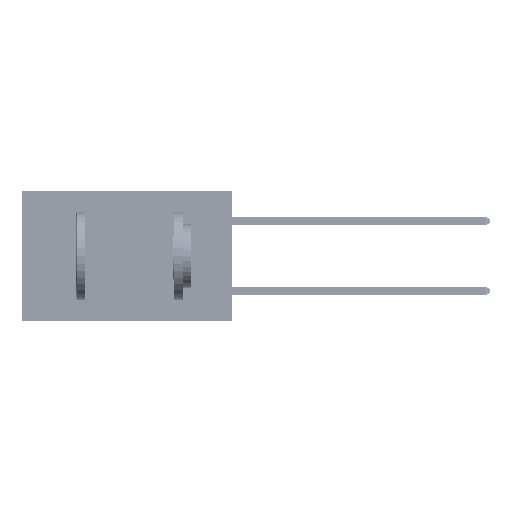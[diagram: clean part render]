
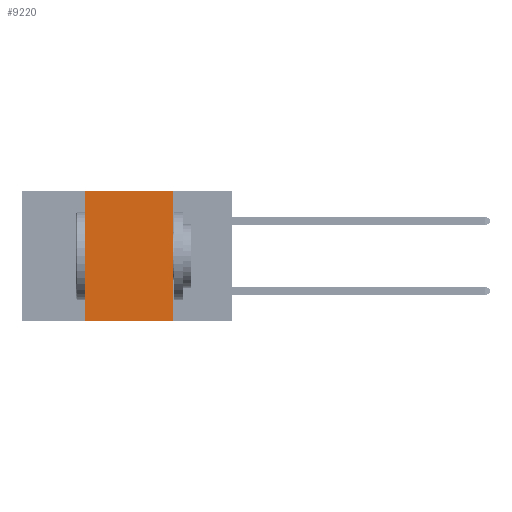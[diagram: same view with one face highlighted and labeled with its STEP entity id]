
A CAD part, left-side view. The second image highlights one B-rep face of the part: STEP entity #9220.
In plain terms, the highlighted planar face has unit normal (-1, 0, 0).
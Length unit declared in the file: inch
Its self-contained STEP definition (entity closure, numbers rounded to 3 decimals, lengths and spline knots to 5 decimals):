
#610 = DIRECTION ( 'NONE',  ( 0., 0., -1. ) ) ;
#2530 = EDGE_CURVE ( 'NONE', #25700, #29957, #48167, .T. ) ;
#3444 = ORIENTED_EDGE ( 'NONE', *, *, #2530, .F. ) ;
#4297 = CARTESIAN_POINT ( 'NONE',  ( 0., 0.17, 0. ) ) ;
#7742 = DIRECTION ( 'NONE',  ( 0., -1., 0. ) ) ;
#7837 = EDGE_CURVE ( 'NONE', #26606, #25754, #17936, .T. ) ;
#9220 = ADVANCED_FACE ( 'NONE', ( #38827 ), #36111, .F. ) ;
#11844 = CARTESIAN_POINT ( 'NONE',  ( 0., 0.6, 0. ) ) ;
#13499 = LINE ( 'NONE', #45412, #21507 ) ;
#13538 = LINE ( 'NONE', #27073, #37643 ) ;
#14273 = CARTESIAN_POINT ( 'NONE',  ( 0., 0.42, 0. ) ) ;
#16411 = CARTESIAN_POINT ( 'NONE',  ( 0., 0.6, 0. ) ) ;
#17936 = LINE ( 'NONE', #32562, #32739 ) ;
#21033 = DIRECTION ( 'NONE',  ( 0., -1., 0. ) ) ;
#21507 = VECTOR ( 'NONE', #33598, 39.37008 ) ;
#25700 = VERTEX_POINT ( 'NONE', #14273 ) ;
#25754 = VERTEX_POINT ( 'NONE', #38962 ) ;
#26606 = VERTEX_POINT ( 'NONE', #27355 ) ;
#27073 = CARTESIAN_POINT ( 'NONE',  ( 0., 0.42, 0. ) ) ;
#27355 = CARTESIAN_POINT ( 'NONE',  ( 0., 0.42, -0.37 ) ) ;
#29957 = VERTEX_POINT ( 'NONE', #4297 ) ;
#31370 = ORIENTED_EDGE ( 'NONE', *, *, #7837, .T. ) ;
#31731 = DIRECTION ( 'NONE',  ( 0., 0., 1. ) ) ;
#32562 = CARTESIAN_POINT ( 'NONE',  ( 0., 0.6, -0.37 ) ) ;
#32739 = VECTOR ( 'NONE', #21033, 39.37008 ) ;
#33598 = DIRECTION ( 'NONE',  ( 0., 0., -1. ) ) ;
#34527 = EDGE_LOOP ( 'NONE', ( #39587, #3444, #43159, #31370 ) ) ;
#35939 = DIRECTION ( 'NONE',  ( 1., 0., 0. ) ) ;
#36111 = PLANE ( 'NONE',  #39441 ) ;
#37605 = VECTOR ( 'NONE', #7742, 39.37008 ) ;
#37643 = VECTOR ( 'NONE', #31731, 39.37008 ) ;
#38827 = FACE_OUTER_BOUND ( 'NONE', #34527, .T. ) ;
#38962 = CARTESIAN_POINT ( 'NONE',  ( 0., 0.17, -0.37 ) ) ;
#39441 = AXIS2_PLACEMENT_3D ( 'NONE', #16411, #35939, #610 ) ;
#39458 = EDGE_CURVE ( 'NONE', #29957, #25754, #13499, .T. ) ;
#39587 = ORIENTED_EDGE ( 'NONE', *, *, #39458, .F. ) ;
#43159 = ORIENTED_EDGE ( 'NONE', *, *, #50444, .F. ) ;
#45412 = CARTESIAN_POINT ( 'NONE',  ( 0., 0.17, 0. ) ) ;
#48167 = LINE ( 'NONE', #11844, #37605 ) ;
#50444 = EDGE_CURVE ( 'NONE', #26606, #25700, #13538, .T. ) ;
